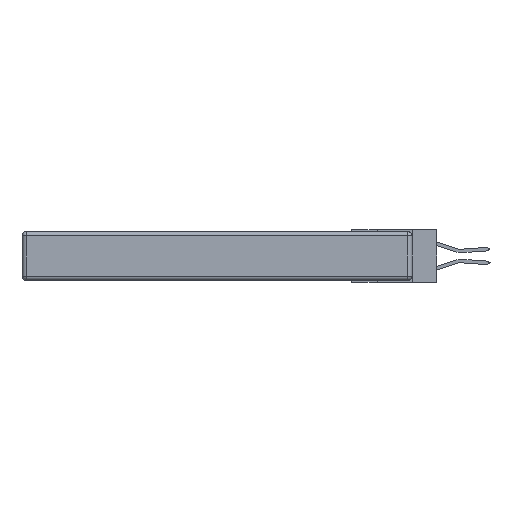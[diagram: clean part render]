
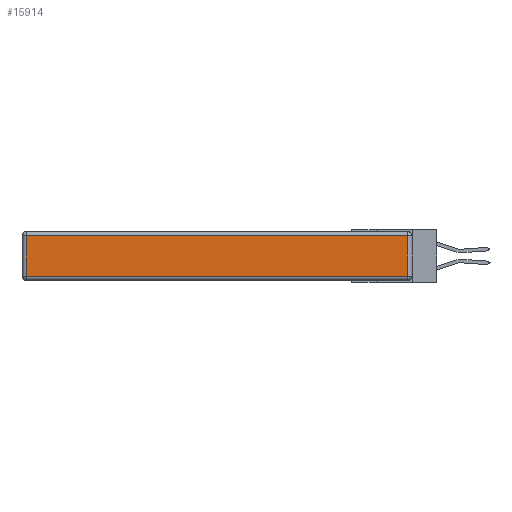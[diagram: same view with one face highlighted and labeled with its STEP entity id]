
A CAD part, left-side view. The second image highlights one B-rep face of the part: STEP entity #15914.
In plain terms, the highlighted planar face has unit normal (-1, 0, 0).
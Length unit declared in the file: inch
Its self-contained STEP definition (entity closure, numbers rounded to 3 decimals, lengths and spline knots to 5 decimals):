
#813 = EDGE_CURVE ( 'NONE', #6392, #8950, #15351, .T. ) ;
#1314 = DIRECTION ( 'NONE',  ( 0., 0., -1. ) ) ;
#1697 = CARTESIAN_POINT ( 'NONE',  ( 0., 0., -0.313 ) ) ;
#1792 = CARTESIAN_POINT ( 'NONE',  ( 0., 2.72, -0.313 ) ) ;
#2052 = VERTEX_POINT ( 'NONE', #1792 ) ;
#2073 = VECTOR ( 'NONE', #1314, 39.37008 ) ;
#2808 = ORIENTED_EDGE ( 'NONE', *, *, #4423, .T. ) ;
#2893 = DIRECTION ( 'NONE',  ( 0., -1., 0. ) ) ;
#3383 = VECTOR ( 'NONE', #11681, 39.37008 ) ;
#3888 = DIRECTION ( 'NONE',  ( -1., 0., 0. ) ) ;
#4423 = EDGE_CURVE ( 'NONE', #8950, #5432, #7351, .T. ) ;
#4782 = DIRECTION ( 'NONE',  ( 0., 1., 0. ) ) ;
#5143 = PLANE ( 'NONE',  #10036 ) ;
#5335 = EDGE_CURVE ( 'NONE', #2052, #6392, #9294, .T. ) ;
#5380 = VECTOR ( 'NONE', #4782, 39.37008 ) ;
#5432 = VERTEX_POINT ( 'NONE', #15321 ) ;
#5953 = VECTOR ( 'NONE', #2893, 39.37008 ) ;
#6392 = VERTEX_POINT ( 'NONE', #8353 ) ;
#7351 = LINE ( 'NONE', #12282, #5380 ) ;
#7799 = ORIENTED_EDGE ( 'NONE', *, *, #813, .T. ) ;
#7900 = EDGE_LOOP ( 'NONE', ( #9392, #7799, #2808, #13766 ) ) ;
#8353 = CARTESIAN_POINT ( 'NONE',  ( 0., 0.03, -0.313 ) ) ;
#8950 = VERTEX_POINT ( 'NONE', #10230 ) ;
#9294 = LINE ( 'NONE', #1697, #5953 ) ;
#9304 = CARTESIAN_POINT ( 'NONE',  ( 0., 0.03, -0.343 ) ) ;
#9392 = ORIENTED_EDGE ( 'NONE', *, *, #5335, .T. ) ;
#9961 = EDGE_CURVE ( 'NONE', #5432, #2052, #13026, .T. ) ;
#10036 = AXIS2_PLACEMENT_3D ( 'NONE', #12785, #3888, #11429 ) ;
#10230 = CARTESIAN_POINT ( 'NONE',  ( 0., 0.03, -0.03 ) ) ;
#11429 = DIRECTION ( 'NONE',  ( 0., 0., 1. ) ) ;
#11681 = DIRECTION ( 'NONE',  ( 0., 0., 1. ) ) ;
#12282 = CARTESIAN_POINT ( 'NONE',  ( 0., 2.75, -0.03 ) ) ;
#12637 = CARTESIAN_POINT ( 'NONE',  ( 0., 2.72, -0.343 ) ) ;
#12785 = CARTESIAN_POINT ( 'NONE',  ( 0., 0., -0.343 ) ) ;
#13026 = LINE ( 'NONE', #12637, #2073 ) ;
#13412 = FACE_OUTER_BOUND ( 'NONE', #7900, .T. ) ;
#13766 = ORIENTED_EDGE ( 'NONE', *, *, #9961, .T. ) ;
#15321 = CARTESIAN_POINT ( 'NONE',  ( 0., 2.72, -0.03 ) ) ;
#15351 = LINE ( 'NONE', #9304, #3383 ) ;
#15914 = ADVANCED_FACE ( 'NONE', ( #13412 ), #5143, .T. ) ;
